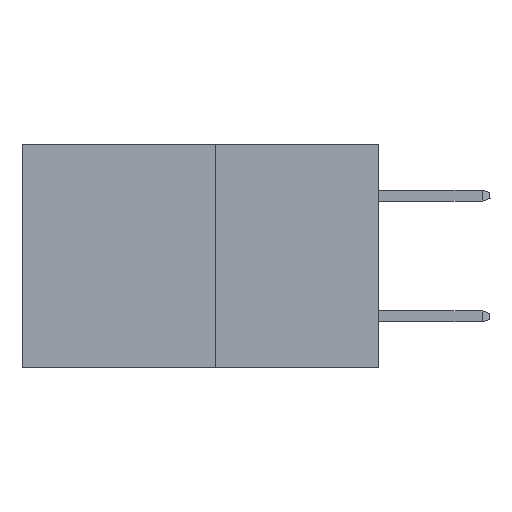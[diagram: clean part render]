
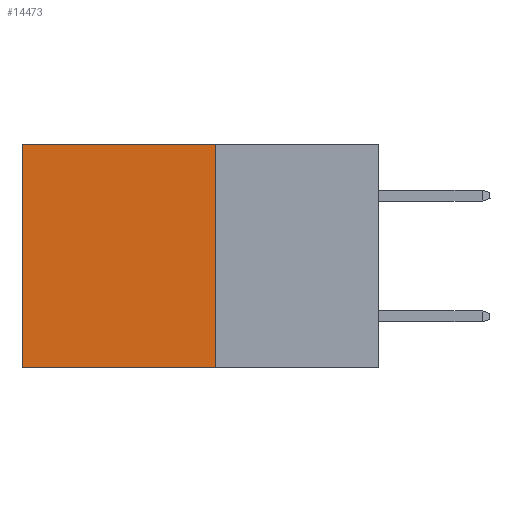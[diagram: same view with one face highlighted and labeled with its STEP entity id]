
A CAD part, left-side view. The second image highlights one B-rep face of the part: STEP entity #14473.
In plain terms, the highlighted planar face has unit normal (-1, 0, 0).
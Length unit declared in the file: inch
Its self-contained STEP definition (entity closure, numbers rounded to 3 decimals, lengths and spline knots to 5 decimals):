
#425 = VECTOR ( 'NONE', #30248, 39.37008 ) ;
#1146 = DIRECTION ( 'NONE',  ( 1., 0., 0. ) ) ;
#1690 = CARTESIAN_POINT ( 'NONE',  ( 0.277, 0.59, -0.37 ) ) ;
#1877 = DIRECTION ( 'NONE',  ( 0., 1., 0. ) ) ;
#2408 = CARTESIAN_POINT ( 'NONE',  ( 0.277, 0.27, -0.37 ) ) ;
#2680 = CARTESIAN_POINT ( 'NONE',  ( 0.277, 0.27, 0. ) ) ;
#5625 = FACE_OUTER_BOUND ( 'NONE', #24192, .T. ) ;
#7328 = ORIENTED_EDGE ( 'NONE', *, *, #10932, .F. ) ;
#10216 = DIRECTION ( 'NONE',  ( 0., 1., 0. ) ) ;
#10672 = LINE ( 'NONE', #2408, #18442 ) ;
#10734 = ORIENTED_EDGE ( 'NONE', *, *, #18119, .F. ) ;
#10932 = EDGE_CURVE ( 'NONE', #12166, #28500, #31593, .T. ) ;
#11622 = PLANE ( 'NONE',  #17625 ) ;
#11980 = EDGE_CURVE ( 'NONE', #12166, #29277, #20680, .T. ) ;
#12166 = VERTEX_POINT ( 'NONE', #2680 ) ;
#12353 = CARTESIAN_POINT ( 'NONE',  ( 0.277, 0.27, 0. ) ) ;
#14473 = ADVANCED_FACE ( 'NONE', ( #5625 ), #11622, .F. ) ;
#16432 = CARTESIAN_POINT ( 'NONE',  ( 0.277, 0.27, -0.37 ) ) ;
#17316 = EDGE_CURVE ( 'NONE', #29277, #33553, #27390, .T. ) ;
#17625 = AXIS2_PLACEMENT_3D ( 'NONE', #32178, #1146, #19485 ) ;
#18119 = EDGE_CURVE ( 'NONE', #28500, #33553, #10672, .T. ) ;
#18442 = VECTOR ( 'NONE', #10216, 39.37008 ) ;
#19485 = DIRECTION ( 'NONE',  ( 0., 0., -1. ) ) ;
#20680 = LINE ( 'NONE', #12353, #32729 ) ;
#23967 = VECTOR ( 'NONE', #28987, 39.37008 ) ;
#24192 = EDGE_LOOP ( 'NONE', ( #28237, #10734, #7328, #32173 ) ) ;
#26407 = CARTESIAN_POINT ( 'NONE',  ( 0.277, 0.27, -0.37 ) ) ;
#27131 = CARTESIAN_POINT ( 'NONE',  ( 0.277, 0.59, 0. ) ) ;
#27390 = LINE ( 'NONE', #1690, #425 ) ;
#28237 = ORIENTED_EDGE ( 'NONE', *, *, #17316, .T. ) ;
#28500 = VERTEX_POINT ( 'NONE', #16432 ) ;
#28987 = DIRECTION ( 'NONE',  ( 0., 0., -1. ) ) ;
#29277 = VERTEX_POINT ( 'NONE', #27131 ) ;
#30248 = DIRECTION ( 'NONE',  ( 0., 0., -1. ) ) ;
#31593 = LINE ( 'NONE', #26407, #23967 ) ;
#32173 = ORIENTED_EDGE ( 'NONE', *, *, #11980, .T. ) ;
#32178 = CARTESIAN_POINT ( 'NONE',  ( 0.277, 0.27, -0.37 ) ) ;
#32729 = VECTOR ( 'NONE', #1877, 39.37008 ) ;
#33553 = VERTEX_POINT ( 'NONE', #33569 ) ;
#33569 = CARTESIAN_POINT ( 'NONE',  ( 0.277, 0.59, -0.37 ) ) ;
